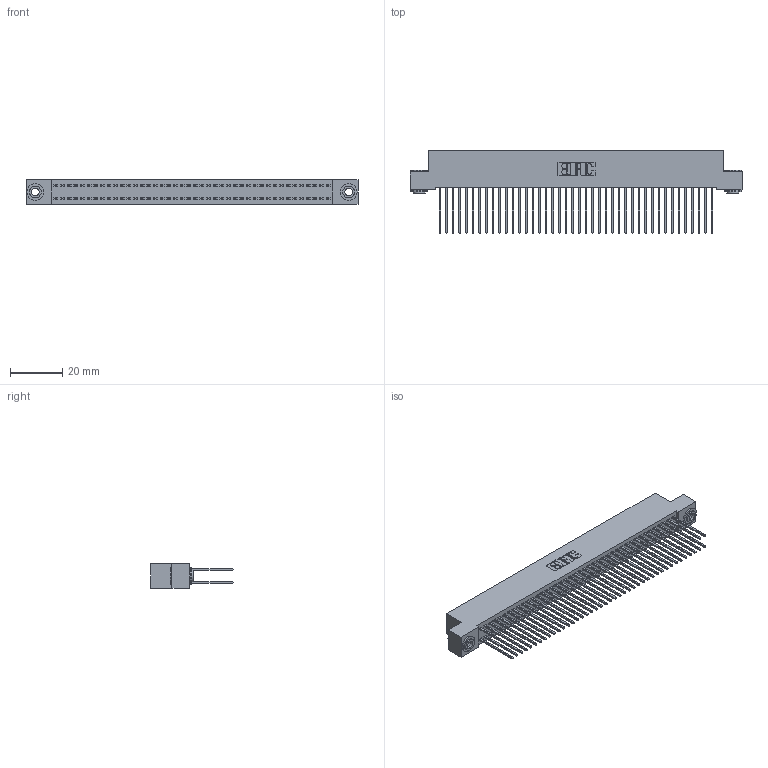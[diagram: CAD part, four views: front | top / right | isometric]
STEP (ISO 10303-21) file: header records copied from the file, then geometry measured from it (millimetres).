
FILE_DESCRIPTION (( 'STEP AP203' ), '1' );
FILE_NAME ('342-084-542-203.STEP', '2018-08-13T17:56:03', ( '' ), ( '' ), 'SwSTEP 2.0', 'SolidWorks 2016', '' );
FILE_SCHEMA (( 'CONFIG_CONTROL_DESIGN' ));
Length unit declared in the file: inch
Products named in the file (4): 342 Part_.156 TH; 345-292-001_345-293-142; 342-250-002_345-250-002-102; 342-084-542-203
Assembly tree (87 placements, depth 2):
  342-084-542-203
    342 Part_.156 TH
    345-292-001_345-293-142  x84
    342-250-002_345-250-002-102  x2
Bounding box: 127 x 31.63 x 9.4 mm (x, y, z)
Volume: 11825.3 mm3; surface area: 21220 mm2
Topology: 87 solids, 87 shells, 4516 faces, 13395 edges, 8814 vertices
Faces by surface type: plane 3100, cylinder 1408, cone 8
Entity records: 27556 total; most frequent: CARTESIAN_POINT 4541, ORIENTED_EDGE 4470, DIRECTION 3913, EDGE_CURVE 2235, VECTOR 2083, LINE 2083, VERTEX_POINT 1486, AXIS2_PLACEMENT_3D 915
